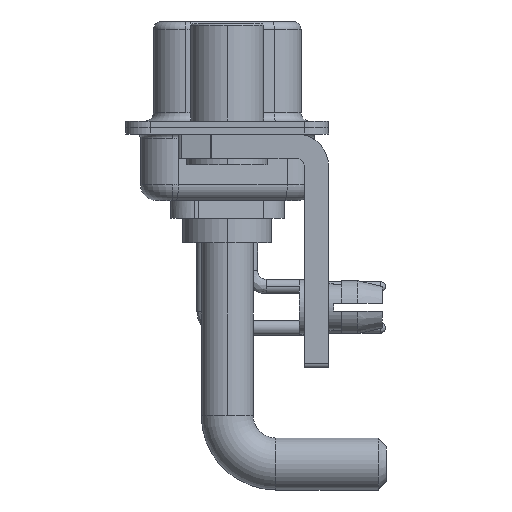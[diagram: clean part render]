
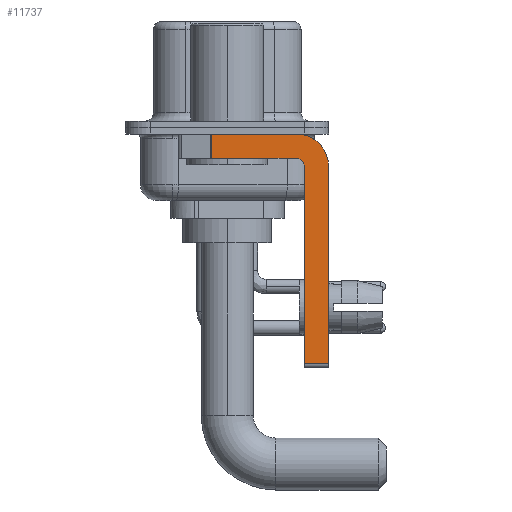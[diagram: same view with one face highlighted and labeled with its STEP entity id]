
A CAD part, left-side view. The second image highlights one B-rep face of the part: STEP entity #11737.
In plain terms, the highlighted planar face has unit normal (-1, 0, 0).
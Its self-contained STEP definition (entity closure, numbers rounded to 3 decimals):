
#1913 = CARTESIAN_POINT ( 'NONE',  ( -2.9, 0.978, -0.4 ) ) ;
#1970 = DIRECTION ( 'NONE',  ( 0., 0., -1. ) ) ;
#2259 = LINE ( 'NONE', #13996, #20105 ) ;
#2575 = DIRECTION ( 'NONE',  ( 0., 1., 0. ) ) ;
#3092 = DIRECTION ( 'NONE',  ( -1., 0., 0. ) ) ;
#3098 = VECTOR ( 'NONE', #5937, 1000. ) ;
#3861 = DIRECTION ( 'NONE',  ( 1., 0., 0. ) ) ;
#3897 = DIRECTION ( 'NONE',  ( 0., -1., 0. ) ) ;
#4080 = VERTEX_POINT ( 'NONE', #23998 ) ;
#4483 = CARTESIAN_POINT ( 'NONE',  ( -2.9, -4.75, -14.55 ) ) ;
#4896 = AXIS2_PLACEMENT_3D ( 'NONE', #23756, #6589, #11265 ) ;
#5203 = AXIS2_PLACEMENT_3D ( 'NONE', #20125, #3092, #17617 ) ;
#5937 = DIRECTION ( 'NONE',  ( 0., 0., 1. ) ) ;
#6046 = CARTESIAN_POINT ( 'NONE',  ( -2.9, -4.25, -1.9 ) ) ;
#6589 = DIRECTION ( 'NONE',  ( 1., 0., 0. ) ) ;
#6603 = EDGE_CURVE ( 'NONE', #25201, #4080, #12961, .T. ) ;
#6924 = EDGE_CURVE ( 'NONE', #25201, #17119, #21388, .T. ) ;
#7212 = CIRCLE ( 'NONE', #5203, 0.5 ) ;
#7250 = EDGE_CURVE ( 'NONE', #7775, #12135, #8717, .T. ) ;
#7437 = AXIS2_PLACEMENT_3D ( 'NONE', #30451, #3861, #20592 ) ;
#7775 = VERTEX_POINT ( 'NONE', #9945 ) ;
#8410 = CIRCLE ( 'NONE', #4896, 2. ) ;
#8717 = LINE ( 'NONE', #25441, #20328 ) ;
#9164 = VERTEX_POINT ( 'NONE', #15103 ) ;
#9668 = CARTESIAN_POINT ( 'NONE',  ( -2.9, -4.25, -14.55 ) ) ;
#9679 = CARTESIAN_POINT ( 'NONE',  ( -2.9, 0.978, -1.9 ) ) ;
#9822 = DIRECTION ( 'NONE',  ( 0., -1., 0. ) ) ;
#9945 = CARTESIAN_POINT ( 'NONE',  ( -2.9, -6.25, -2.4 ) ) ;
#11190 = EDGE_CURVE ( 'NONE', #4080, #7775, #8410, .T. ) ;
#11219 = FACE_OUTER_BOUND ( 'NONE', #18368, .T. ) ;
#11265 = DIRECTION ( 'NONE',  ( 0., 0., -1. ) ) ;
#11737 = ADVANCED_FACE ( 'NONE', ( #11219 ), #25290, .F. ) ;
#12135 = VERTEX_POINT ( 'NONE', #14553 ) ;
#12603 = EDGE_CURVE ( 'NONE', #25565, #12135, #19505, .T. ) ;
#12961 = LINE ( 'NONE', #25319, #16797 ) ;
#13996 = CARTESIAN_POINT ( 'NONE',  ( -2.9, -4.25, -1.9 ) ) ;
#14130 = ORIENTED_EDGE ( 'NONE', *, *, #6603, .F. ) ;
#14553 = CARTESIAN_POINT ( 'NONE',  ( -2.9, -6.25, -14.55 ) ) ;
#14842 = CARTESIAN_POINT ( 'NONE',  ( -2.9, -4.75, -14.8 ) ) ;
#15103 = CARTESIAN_POINT ( 'NONE',  ( -2.9, -4.75, -2.4 ) ) ;
#15307 = VECTOR ( 'NONE', #17003, 1000. ) ;
#15451 = VECTOR ( 'NONE', #9822, 1000. ) ;
#16189 = ORIENTED_EDGE ( 'NONE', *, *, #11190, .F. ) ;
#16797 = VECTOR ( 'NONE', #3897, 1000. ) ;
#16896 = ORIENTED_EDGE ( 'NONE', *, *, #6924, .T. ) ;
#17003 = DIRECTION ( 'NONE',  ( 0., 0., -1. ) ) ;
#17119 = VERTEX_POINT ( 'NONE', #9679 ) ;
#17617 = DIRECTION ( 'NONE',  ( 0., 0., 1. ) ) ;
#18368 = EDGE_LOOP ( 'NONE', ( #14130, #16896, #27367, #23537, #25033, #20635, #28363, #16189 ) ) ;
#18645 = EDGE_CURVE ( 'NONE', #25565, #9164, #27037, .T. ) ;
#19385 = EDGE_CURVE ( 'NONE', #24018, #17119, #2259, .T. ) ;
#19505 = LINE ( 'NONE', #9668, #15451 ) ;
#20105 = VECTOR ( 'NONE', #2575, 1000. ) ;
#20125 = CARTESIAN_POINT ( 'NONE',  ( -2.9, -4.25, -2.4 ) ) ;
#20328 = VECTOR ( 'NONE', #1970, 1000. ) ;
#20592 = DIRECTION ( 'NONE',  ( 0., 0., -1. ) ) ;
#20635 = ORIENTED_EDGE ( 'NONE', *, *, #12603, .T. ) ;
#20893 = EDGE_CURVE ( 'NONE', #9164, #24018, #7212, .T. ) ;
#21388 = LINE ( 'NONE', #28893, #15307 ) ;
#23537 = ORIENTED_EDGE ( 'NONE', *, *, #20893, .F. ) ;
#23756 = CARTESIAN_POINT ( 'NONE',  ( -2.9, -4.25, -2.4 ) ) ;
#23998 = CARTESIAN_POINT ( 'NONE',  ( -2.9, -4.25, -0.4 ) ) ;
#24018 = VERTEX_POINT ( 'NONE', #6046 ) ;
#25033 = ORIENTED_EDGE ( 'NONE', *, *, #18645, .F. ) ;
#25201 = VERTEX_POINT ( 'NONE', #1913 ) ;
#25290 = PLANE ( 'NONE',  #7437 ) ;
#25319 = CARTESIAN_POINT ( 'NONE',  ( -2.9, 3., -0.4 ) ) ;
#25441 = CARTESIAN_POINT ( 'NONE',  ( -2.9, -6.25, -2.4 ) ) ;
#25565 = VERTEX_POINT ( 'NONE', #4483 ) ;
#27037 = LINE ( 'NONE', #14842, #3098 ) ;
#27367 = ORIENTED_EDGE ( 'NONE', *, *, #19385, .F. ) ;
#28363 = ORIENTED_EDGE ( 'NONE', *, *, #7250, .F. ) ;
#28893 = CARTESIAN_POINT ( 'NONE',  ( -2.9, 0.978, -1.9 ) ) ;
#30451 = CARTESIAN_POINT ( 'NONE',  ( -2.9, -4.25, -2.4 ) ) ;
